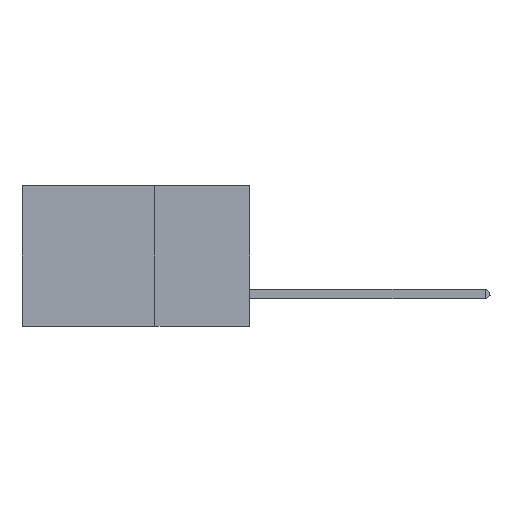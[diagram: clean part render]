
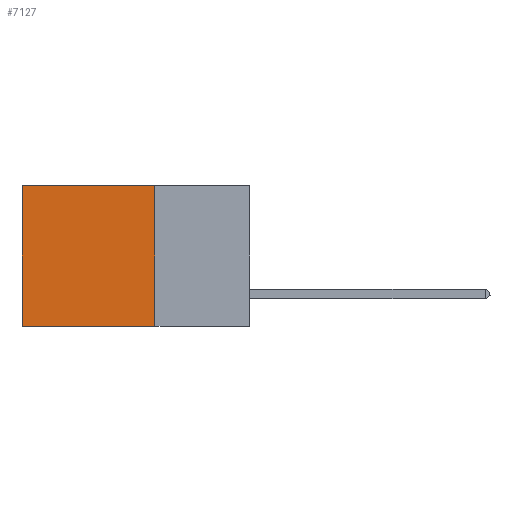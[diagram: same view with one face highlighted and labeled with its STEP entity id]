
A CAD part, left-side view. The second image highlights one B-rep face of the part: STEP entity #7127.
In plain terms, the highlighted planar face has unit normal (-1, 0, 0).
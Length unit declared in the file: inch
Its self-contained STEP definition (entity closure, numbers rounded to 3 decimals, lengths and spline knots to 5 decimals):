
#35 = VECTOR ( 'NONE', #17183, 39.37008 ) ;
#238 = EDGE_CURVE ( 'NONE', #1397, #14710, #686, .T. ) ;
#354 = CARTESIAN_POINT ( 'NONE',  ( 0.2875, 0.6, -0.37 ) ) ;
#686 = LINE ( 'NONE', #10495, #13516 ) ;
#1397 = VERTEX_POINT ( 'NONE', #5651 ) ;
#2709 = EDGE_CURVE ( 'NONE', #6546, #14706, #6568, .T. ) ;
#3701 = CARTESIAN_POINT ( 'NONE',  ( 0.2875, 0.25, -0.37 ) ) ;
#4299 = CARTESIAN_POINT ( 'NONE',  ( 0.2875, 0.25, 0. ) ) ;
#4785 = ORIENTED_EDGE ( 'NONE', *, *, #8645, .F. ) ;
#5518 = CARTESIAN_POINT ( 'NONE',  ( 0.2875, 0.25, -0.37 ) ) ;
#5651 = CARTESIAN_POINT ( 'NONE',  ( 0.2875, 0.25, 0. ) ) ;
#5846 = LINE ( 'NONE', #5518, #35 ) ;
#6322 = VECTOR ( 'NONE', #7857, 39.37008 ) ;
#6461 = LINE ( 'NONE', #4299, #16911 ) ;
#6546 = VERTEX_POINT ( 'NONE', #7033 ) ;
#6568 = LINE ( 'NONE', #14712, #6322 ) ;
#7033 = CARTESIAN_POINT ( 'NONE',  ( 0.2875, 0.6, 0. ) ) ;
#7127 = ADVANCED_FACE ( 'NONE', ( #17663 ), #13597, .F. ) ;
#7857 = DIRECTION ( 'NONE',  ( 0., 0., -1. ) ) ;
#8645 = EDGE_CURVE ( 'NONE', #14710, #14706, #5846, .T. ) ;
#8786 = DIRECTION ( 'NONE',  ( 0., 0., -1. ) ) ;
#10495 = CARTESIAN_POINT ( 'NONE',  ( 0.2875, 0.25, 0. ) ) ;
#10555 = ORIENTED_EDGE ( 'NONE', *, *, #2709, .T. ) ;
#10685 = AXIS2_PLACEMENT_3D ( 'NONE', #11999, #16936, #8786 ) ;
#11403 = ORIENTED_EDGE ( 'NONE', *, *, #238, .F. ) ;
#11999 = CARTESIAN_POINT ( 'NONE',  ( 0.2875, 0.25, 0. ) ) ;
#13516 = VECTOR ( 'NONE', #18746, 39.37008 ) ;
#13597 = PLANE ( 'NONE',  #10685 ) ;
#14706 = VERTEX_POINT ( 'NONE', #354 ) ;
#14710 = VERTEX_POINT ( 'NONE', #3701 ) ;
#14712 = CARTESIAN_POINT ( 'NONE',  ( 0.2875, 0.6, 0. ) ) ;
#15887 = ORIENTED_EDGE ( 'NONE', *, *, #17855, .T. ) ;
#16086 = DIRECTION ( 'NONE',  ( 0., 1., 0. ) ) ;
#16390 = EDGE_LOOP ( 'NONE', ( #10555, #4785, #11403, #15887 ) ) ;
#16911 = VECTOR ( 'NONE', #16086, 39.37008 ) ;
#16936 = DIRECTION ( 'NONE',  ( 1., 0., 0. ) ) ;
#17183 = DIRECTION ( 'NONE',  ( 0., 1., 0. ) ) ;
#17663 = FACE_OUTER_BOUND ( 'NONE', #16390, .T. ) ;
#17855 = EDGE_CURVE ( 'NONE', #1397, #6546, #6461, .T. ) ;
#18746 = DIRECTION ( 'NONE',  ( 0., 0., -1. ) ) ;
